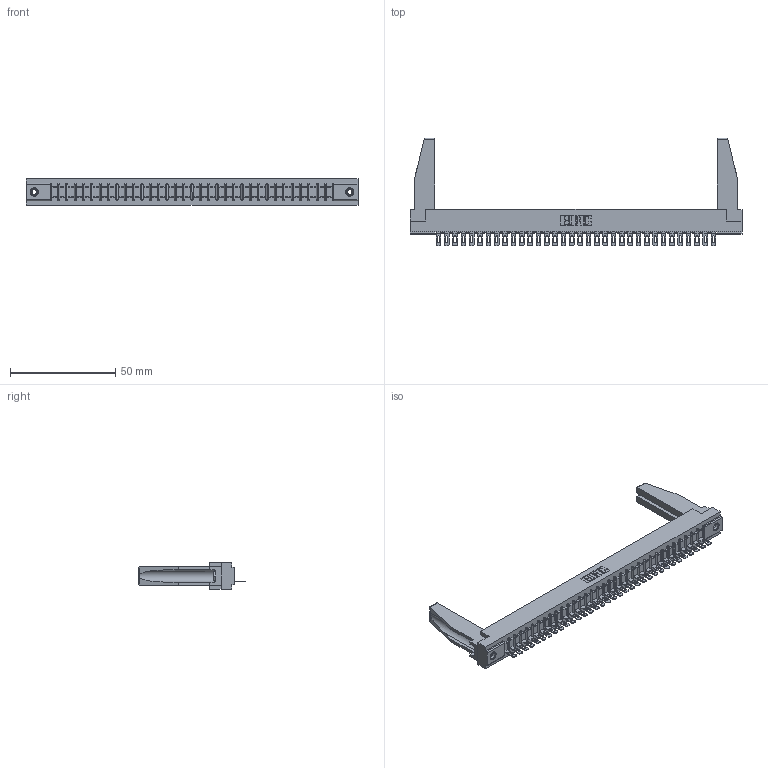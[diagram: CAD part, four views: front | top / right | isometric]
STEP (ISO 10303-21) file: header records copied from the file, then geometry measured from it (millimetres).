
FILE_DESCRIPTION (( 'STEP AP203' ), '1' );
FILE_NAME ('307-034-401-178.STEP', '2020-09-28T21:13:31', ( '' ), ( '' ), 'SwSTEP 2.0', 'SolidWorks 2020', '' );
FILE_SCHEMA (( 'CONFIG_CONTROL_DESIGN' ));
Length unit declared in the file: inch
Products named in the file (5): 307-290-002_501; 307-220-078; 307 Part_.156 Dia Mounting Holes; 307-034-401-178; 345-250-001_345-250-001-102
Assembly tree (39 placements, depth 2):
  307-034-401-178
    307 Part_.156 Dia Mounting Holes
    307-290-002_501  x34
    307-220-078  x2
    345-250-001_345-250-001-102  x2
Bounding box: 157.73 x 51.13 x 12.7 mm (x, y, z)
Volume: 20842.8 mm3; surface area: 25065.7 mm2
Topology: 39 solids, 39 shells, 2867 faces, 8745 edges, 5726 vertices
Faces by surface type: plane 1650, cylinder 1131, sphere 70, cone 12, torus 4
Entity records: 33367 total; most frequent: CARTESIAN_POINT 5626, ORIENTED_EDGE 5572, DIRECTION 5430, EDGE_CURVE 2786, LINE 2130, VECTOR 2130, VERTEX_POINT 1804, AXIS2_PLACEMENT_3D 1650
